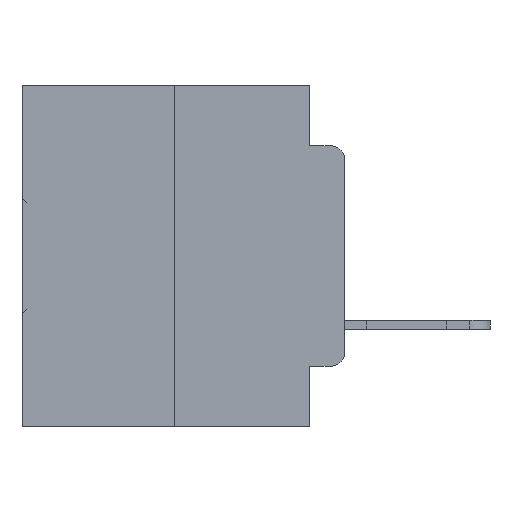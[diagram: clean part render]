
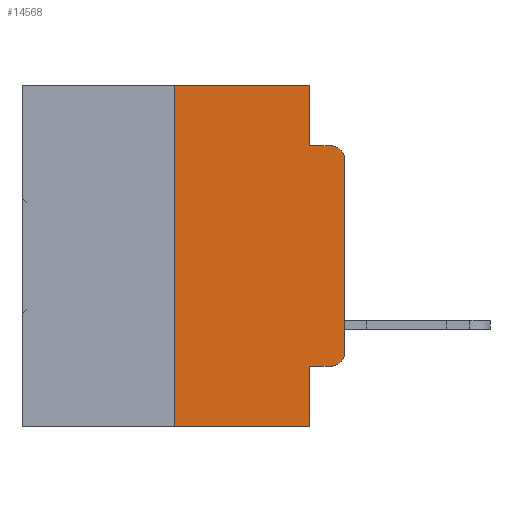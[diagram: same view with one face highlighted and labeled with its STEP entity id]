
A CAD part, left-side view. The second image highlights one B-rep face of the part: STEP entity #14568.
In plain terms, the highlighted planar face has unit normal (-1, 0, 0).
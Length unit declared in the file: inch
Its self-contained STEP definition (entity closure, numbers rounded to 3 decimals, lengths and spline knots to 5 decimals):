
#28 = CARTESIAN_POINT ( 'NONE',  ( 0., 0.051, -0.0885 ) ) ;
#427 = FACE_OUTER_BOUND ( 'NONE', #20119, .T. ) ;
#447 = DIRECTION ( 'NONE',  ( 0., 0., -1. ) ) ;
#855 = LINE ( 'NONE', #11645, #21159 ) ;
#1908 = LINE ( 'NONE', #19823, #33354 ) ;
#1998 = CARTESIAN_POINT ( 'NONE',  ( 0., 0., -0.3915 ) ) ;
#2385 = EDGE_CURVE ( 'NONE', #18757, #22866, #19886, .T. ) ;
#3040 = VERTEX_POINT ( 'NONE', #26594 ) ;
#3070 = EDGE_CURVE ( 'NONE', #30807, #4522, #17479, .T. ) ;
#3235 = DIRECTION ( 'NONE',  ( 0., -1., 0. ) ) ;
#4350 = VECTOR ( 'NONE', #20434, 39.37008 ) ;
#4522 = VERTEX_POINT ( 'NONE', #21677 ) ;
#4546 = EDGE_CURVE ( 'NONE', #29599, #8364, #1908, .T. ) ;
#4568 = CARTESIAN_POINT ( 'NONE',  ( 0., 0.02, -0.4115 ) ) ;
#5376 = CARTESIAN_POINT ( 'NONE',  ( 0., 0.051, 0. ) ) ;
#6074 = EDGE_CURVE ( 'NONE', #3040, #18757, #855, .T. ) ;
#6657 = VERTEX_POINT ( 'NONE', #28058 ) ;
#6816 = DIRECTION ( 'NONE',  ( 0., 0., -1. ) ) ;
#6863 = CARTESIAN_POINT ( 'NONE',  ( 0., 0.051, -0.0885 ) ) ;
#7003 = VECTOR ( 'NONE', #21767, 39.37008 ) ;
#7759 = VECTOR ( 'NONE', #3235, 39.37008 ) ;
#8350 = VECTOR ( 'NONE', #6816, 39.37008 ) ;
#8364 = VERTEX_POINT ( 'NONE', #10403 ) ;
#9011 = EDGE_CURVE ( 'NONE', #24787, #14899, #13992, .T. ) ;
#9180 = LINE ( 'NONE', #5376, #8350 ) ;
#9731 = CARTESIAN_POINT ( 'NONE',  ( 0., 0.02, -0.0885 ) ) ;
#10403 = CARTESIAN_POINT ( 'NONE',  ( 0., 0., -0.1085 ) ) ;
#11412 = EDGE_CURVE ( 'NONE', #30807, #6657, #29942, .T. ) ;
#11645 = CARTESIAN_POINT ( 'NONE',  ( 0., 0.051, 0. ) ) ;
#11782 = DIRECTION ( 'NONE',  ( 0., 0., -1. ) ) ;
#12542 = EDGE_CURVE ( 'NONE', #14899, #29599, #13767, .T. ) ;
#12558 = CARTESIAN_POINT ( 'NONE',  ( 0., 0.051, -0.4115 ) ) ;
#13331 = AXIS2_PLACEMENT_3D ( 'NONE', #16562, #16470, #16448 ) ;
#13767 = CIRCLE ( 'NONE', #26211, 0.02 ) ;
#13992 = LINE ( 'NONE', #21971, #7003 ) ;
#14568 = ADVANCED_FACE ( 'NONE', ( #427 ), #16552, .F. ) ;
#14882 = EDGE_CURVE ( 'NONE', #24787, #4522, #9180, .T. ) ;
#14899 = VERTEX_POINT ( 'NONE', #4568 ) ;
#15311 = DIRECTION ( 'NONE',  ( 0., 0., -1. ) ) ;
#15351 = DIRECTION ( 'NONE',  ( -1., 0., 0. ) ) ;
#15425 = CARTESIAN_POINT ( 'NONE',  ( 0., 0.02, -0.3915 ) ) ;
#16190 = CARTESIAN_POINT ( 'NONE',  ( 0., 0.473, -0.5 ) ) ;
#16448 = DIRECTION ( 'NONE',  ( 0., 0., -1. ) ) ;
#16470 = DIRECTION ( 'NONE',  ( 1., 0., 0. ) ) ;
#16552 = PLANE ( 'NONE',  #13331 ) ;
#16562 = CARTESIAN_POINT ( 'NONE',  ( 0., 0.473, 0. ) ) ;
#16666 = DIRECTION ( 'NONE',  ( -1., 0., 0. ) ) ;
#17348 = ORIENTED_EDGE ( 'NONE', *, *, #29990, .T. ) ;
#17439 = ORIENTED_EDGE ( 'NONE', *, *, #4546, .T. ) ;
#17479 = LINE ( 'NONE', #16190, #30663 ) ;
#17487 = CIRCLE ( 'NONE', #17499, 0.02 ) ;
#17499 = AXIS2_PLACEMENT_3D ( 'NONE', #31469, #16666, #447 ) ;
#17526 = ORIENTED_EDGE ( 'NONE', *, *, #2385, .F. ) ;
#17742 = ORIENTED_EDGE ( 'NONE', *, *, #22232, .F. ) ;
#17961 = ORIENTED_EDGE ( 'NONE', *, *, #11412, .F. ) ;
#18238 = ORIENTED_EDGE ( 'NONE', *, *, #3070, .T. ) ;
#18298 = ORIENTED_EDGE ( 'NONE', *, *, #9011, .T. ) ;
#18326 = ORIENTED_EDGE ( 'NONE', *, *, #14882, .F. ) ;
#18645 = ORIENTED_EDGE ( 'NONE', *, *, #12542, .T. ) ;
#18757 = VERTEX_POINT ( 'NONE', #28 ) ;
#18831 = VECTOR ( 'NONE', #20688, 39.37008 ) ;
#19823 = CARTESIAN_POINT ( 'NONE',  ( 0., 0., 0. ) ) ;
#19886 = LINE ( 'NONE', #6863, #7759 ) ;
#20119 = EDGE_LOOP ( 'NONE', ( #17439, #17348, #17526, #23692, #17742, #17961, #18238, #18326, #18298, #18645 ) ) ;
#20434 = DIRECTION ( 'NONE',  ( 0., 0., 1. ) ) ;
#20540 = CARTESIAN_POINT ( 'NONE',  ( 0., 0.25, 0. ) ) ;
#20688 = DIRECTION ( 'NONE',  ( 0., -1., 0. ) ) ;
#20729 = CARTESIAN_POINT ( 'NONE',  ( 0., 0.473, 0. ) ) ;
#20814 = DIRECTION ( 'NONE',  ( 0., 0., 1. ) ) ;
#21159 = VECTOR ( 'NONE', #11782, 39.37008 ) ;
#21677 = CARTESIAN_POINT ( 'NONE',  ( 0., 0.051, -0.5 ) ) ;
#21767 = DIRECTION ( 'NONE',  ( 0., -1., 0. ) ) ;
#21971 = CARTESIAN_POINT ( 'NONE',  ( 0., 0.051, -0.4115 ) ) ;
#22232 = EDGE_CURVE ( 'NONE', #6657, #3040, #31921, .T. ) ;
#22866 = VERTEX_POINT ( 'NONE', #9731 ) ;
#23692 = ORIENTED_EDGE ( 'NONE', *, *, #6074, .F. ) ;
#24787 = VERTEX_POINT ( 'NONE', #12558 ) ;
#26007 = DIRECTION ( 'NONE',  ( 0., -1., 0. ) ) ;
#26211 = AXIS2_PLACEMENT_3D ( 'NONE', #15425, #15351, #15311 ) ;
#26594 = CARTESIAN_POINT ( 'NONE',  ( 0., 0.051, 0. ) ) ;
#28058 = CARTESIAN_POINT ( 'NONE',  ( 0., 0.25, 0. ) ) ;
#29599 = VERTEX_POINT ( 'NONE', #1998 ) ;
#29942 = LINE ( 'NONE', #20540, #4350 ) ;
#29990 = EDGE_CURVE ( 'NONE', #8364, #22866, #17487, .T. ) ;
#30663 = VECTOR ( 'NONE', #26007, 39.37008 ) ;
#30807 = VERTEX_POINT ( 'NONE', #30828 ) ;
#30828 = CARTESIAN_POINT ( 'NONE',  ( 0., 0.25, -0.5 ) ) ;
#31469 = CARTESIAN_POINT ( 'NONE',  ( 0., 0.02, -0.1085 ) ) ;
#31921 = LINE ( 'NONE', #20729, #18831 ) ;
#33354 = VECTOR ( 'NONE', #20814, 39.37008 ) ;
